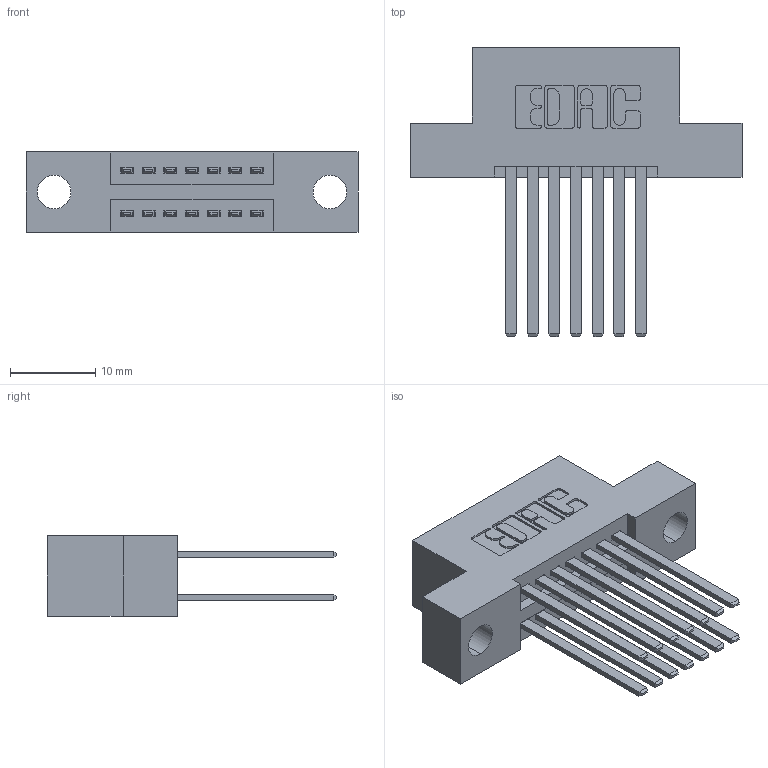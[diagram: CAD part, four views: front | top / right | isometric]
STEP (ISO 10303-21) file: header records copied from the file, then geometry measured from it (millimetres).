
FILE_DESCRIPTION (( 'STEP AP203' ), '1' );
FILE_NAME ('345-014-544-204.STEP', '2018-08-18T17:34:56', ( '' ), ( '' ), 'SwSTEP 2.0', 'SolidWorks 2016', '' );
FILE_SCHEMA (( 'CONFIG_CONTROL_DESIGN' ));
Length unit declared in the file: inch
Products named in the file (3): 345 Part_Flush Mounting Lugs - 0.156 Dia-TH; 345-292-001_345-293-144; 345-014-544-204
Assembly tree (15 placements, depth 2):
  345-014-544-204
    345 Part_Flush Mounting Lugs - 0.156 Dia-TH
    345-292-001_345-293-144  x14
Bounding box: 38.99 x 33.96 x 9.4 mm (x, y, z)
Volume: 3570.9 mm3; surface area: 4991 mm2
Topology: 15 solids, 15 shells, 742 faces, 2175 edges, 1430 vertices
Faces by surface type: plane 486, cylinder 256
Entity records: 10023 total; most frequent: CARTESIAN_POINT 1712, ORIENTED_EDGE 1646, DIRECTION 1551, EDGE_CURVE 823, VECTOR 667, LINE 667, VERTEX_POINT 546, AXIS2_PLACEMENT_3D 442
